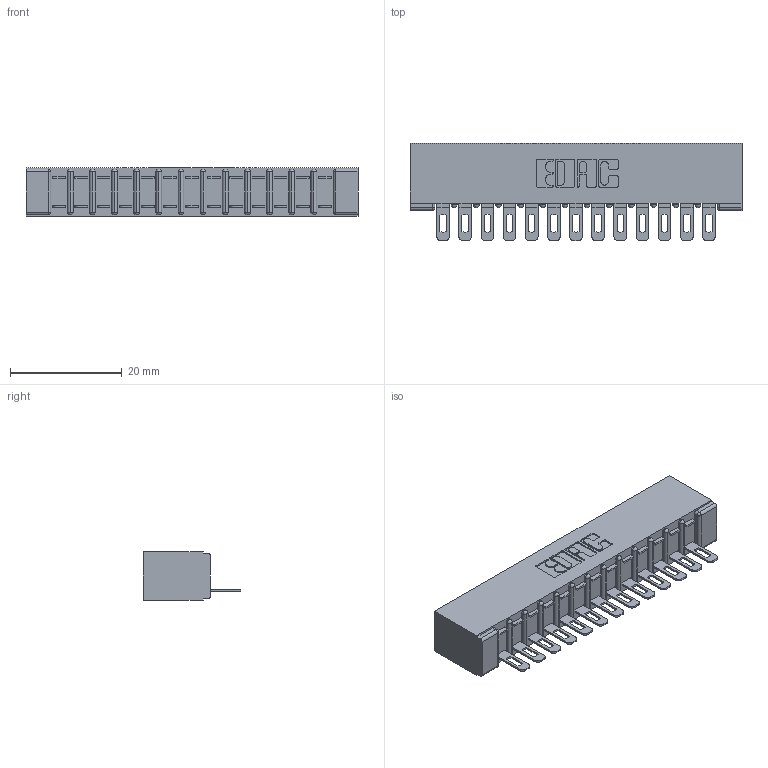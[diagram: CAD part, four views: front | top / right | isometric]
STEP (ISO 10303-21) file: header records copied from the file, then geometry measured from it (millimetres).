
FILE_DESCRIPTION (( 'STEP AP203' ), '1' );
FILE_NAME ('307-013-501-101.STEP', '2019-09-04T20:03:43', ( '' ), ( '' ), 'SwSTEP 2.0', 'SolidWorks 2016', '' );
FILE_SCHEMA (( 'CONFIG_CONTROL_DESIGN' ));
Length unit declared in the file: inch
Products named in the file (3): 307 Part_No Mounting Lugs; 307-290-002_501; 307-013-501-101
Assembly tree (14 placements, depth 2):
  307-013-501-101
    307 Part_No Mounting Lugs
    307-290-002_501  x13
Bounding box: 59.39 x 17.42 x 8.71 mm (x, y, z)
Volume: 4169.4 mm3; surface area: 7677.8 mm2
Topology: 14 solids, 14 shells, 1112 faces, 3393 edges, 2222 vertices
Faces by surface type: plane 638, cylinder 446, sphere 28
Entity records: 15236 total; most frequent: CARTESIAN_POINT 2564, ORIENTED_EDGE 2554, DIRECTION 2507, EDGE_CURVE 1277, VECTOR 961, LINE 961, VERTEX_POINT 830, AXIS2_PLACEMENT_3D 773
